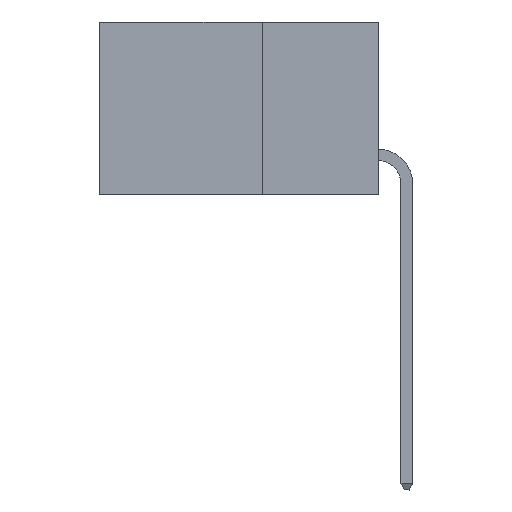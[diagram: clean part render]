
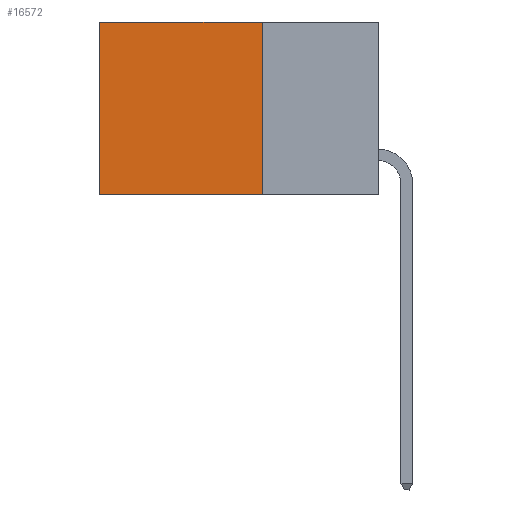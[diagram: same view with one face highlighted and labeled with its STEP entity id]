
A CAD part, left-side view. The second image highlights one B-rep face of the part: STEP entity #16572.
In plain terms, the highlighted planar face has unit normal (-1, 0, 0).
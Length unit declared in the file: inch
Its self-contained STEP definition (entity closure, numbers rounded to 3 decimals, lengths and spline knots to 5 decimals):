
#68 = DIRECTION ( 'NONE',  ( 1., 0., 0. ) ) ;
#1922 = DIRECTION ( 'NONE',  ( 0., 0., -1. ) ) ;
#2201 = LINE ( 'NONE', #13535, #13216 ) ;
#3420 = ORIENTED_EDGE ( 'NONE', *, *, #20381, .T. ) ;
#3865 = EDGE_CURVE ( 'NONE', #19198, #14286, #9035, .T. ) ;
#3968 = EDGE_CURVE ( 'NONE', #8631, #14243, #20295, .T. ) ;
#7895 = CARTESIAN_POINT ( 'NONE',  ( 0.298, 0.6, 0. ) ) ;
#8452 = VECTOR ( 'NONE', #9756, 39.37008 ) ;
#8631 = VERTEX_POINT ( 'NONE', #19264 ) ;
#9035 = LINE ( 'NONE', #7895, #8452 ) ;
#9538 = ORIENTED_EDGE ( 'NONE', *, *, #3968, .F. ) ;
#9756 = DIRECTION ( 'NONE',  ( 0., 0., -1. ) ) ;
#10313 = CARTESIAN_POINT ( 'NONE',  ( 0.298, 0.25, -0.37 ) ) ;
#10438 = VECTOR ( 'NONE', #18119, 39.37008 ) ;
#11141 = ORIENTED_EDGE ( 'NONE', *, *, #11893, .F. ) ;
#11893 = EDGE_CURVE ( 'NONE', #14243, #14286, #2201, .T. ) ;
#13185 = PLANE ( 'NONE',  #14232 ) ;
#13216 = VECTOR ( 'NONE', #19167, 39.37008 ) ;
#13535 = CARTESIAN_POINT ( 'NONE',  ( 0.298, 0.25, -0.37 ) ) ;
#13628 = CARTESIAN_POINT ( 'NONE',  ( 0.298, 0.25, 0. ) ) ;
#13827 = ORIENTED_EDGE ( 'NONE', *, *, #3865, .T. ) ;
#14001 = VECTOR ( 'NONE', #15593, 39.37008 ) ;
#14232 = AXIS2_PLACEMENT_3D ( 'NONE', #20367, #68, #1922 ) ;
#14243 = VERTEX_POINT ( 'NONE', #10313 ) ;
#14286 = VERTEX_POINT ( 'NONE', #19611 ) ;
#15064 = CARTESIAN_POINT ( 'NONE',  ( 0.298, 0.6, 0. ) ) ;
#15593 = DIRECTION ( 'NONE',  ( 0., 1., 0. ) ) ;
#15627 = EDGE_LOOP ( 'NONE', ( #13827, #11141, #9538, #3420 ) ) ;
#16572 = ADVANCED_FACE ( 'NONE', ( #19336 ), #13185, .F. ) ;
#16924 = LINE ( 'NONE', #13628, #14001 ) ;
#18119 = DIRECTION ( 'NONE',  ( 0., 0., -1. ) ) ;
#19167 = DIRECTION ( 'NONE',  ( 0., 1., 0. ) ) ;
#19198 = VERTEX_POINT ( 'NONE', #15064 ) ;
#19264 = CARTESIAN_POINT ( 'NONE',  ( 0.298, 0.25, 0. ) ) ;
#19336 = FACE_OUTER_BOUND ( 'NONE', #15627, .T. ) ;
#19611 = CARTESIAN_POINT ( 'NONE',  ( 0.298, 0.6, -0.37 ) ) ;
#20295 = LINE ( 'NONE', #21936, #10438 ) ;
#20367 = CARTESIAN_POINT ( 'NONE',  ( 0.298, 0.25, 0. ) ) ;
#20381 = EDGE_CURVE ( 'NONE', #8631, #19198, #16924, .T. ) ;
#21936 = CARTESIAN_POINT ( 'NONE',  ( 0.298, 0.25, 0. ) ) ;
